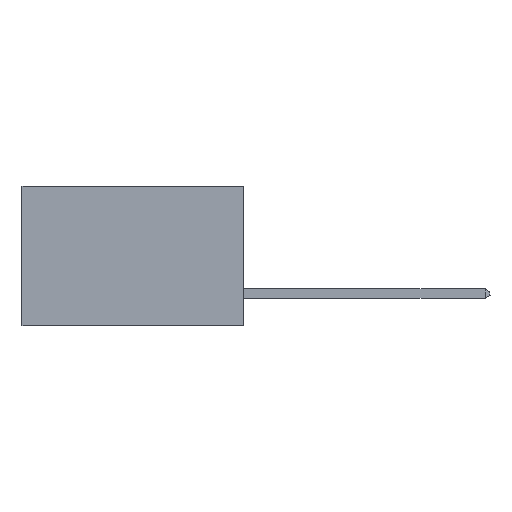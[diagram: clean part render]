
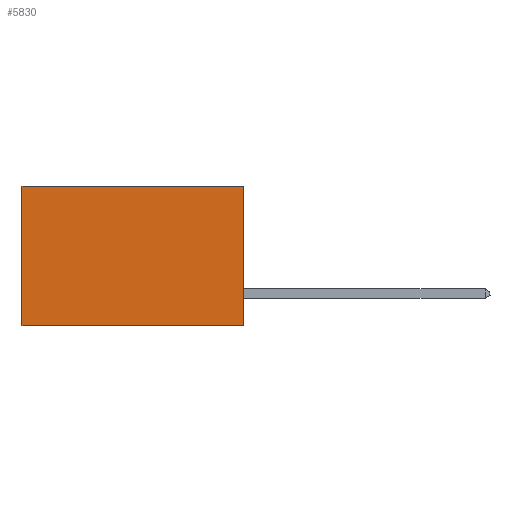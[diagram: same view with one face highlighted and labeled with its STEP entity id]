
A CAD part, left-side view. The second image highlights one B-rep face of the part: STEP entity #5830.
In plain terms, the highlighted planar face has unit normal (-1, 0, 0).
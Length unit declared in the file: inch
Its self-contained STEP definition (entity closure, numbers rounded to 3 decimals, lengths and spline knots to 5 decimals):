
#313 = VERTEX_POINT ( 'NONE', #10428 ) ;
#1306 = EDGE_LOOP ( 'NONE', ( #21295, #5080, #8119, #3326 ) ) ;
#1521 = VECTOR ( 'NONE', #9994, 39.37008 ) ;
#2545 = CARTESIAN_POINT ( 'NONE',  ( 0.277, 0.59, -0.37 ) ) ;
#3247 = CARTESIAN_POINT ( 'NONE',  ( 0.277, 0., 0. ) ) ;
#3326 = ORIENTED_EDGE ( 'NONE', *, *, #8300, .T. ) ;
#4000 = VECTOR ( 'NONE', #4506, 39.37008 ) ;
#4055 = EDGE_CURVE ( 'NONE', #6846, #10834, #22341, .T. ) ;
#4356 = CARTESIAN_POINT ( 'NONE',  ( 0.277, 0., -0.37 ) ) ;
#4506 = DIRECTION ( 'NONE',  ( 0., 0., -1. ) ) ;
#5080 = ORIENTED_EDGE ( 'NONE', *, *, #6585, .F. ) ;
#5112 = FACE_OUTER_BOUND ( 'NONE', #1306, .T. ) ;
#5409 = AXIS2_PLACEMENT_3D ( 'NONE', #12770, #12705, #12666 ) ;
#5830 = ADVANCED_FACE ( 'NONE', ( #5112 ), #13014, .F. ) ;
#6585 = EDGE_CURVE ( 'NONE', #10834, #313, #7511, .T. ) ;
#6846 = VERTEX_POINT ( 'NONE', #3247 ) ;
#7511 = LINE ( 'NONE', #11768, #22531 ) ;
#8119 = ORIENTED_EDGE ( 'NONE', *, *, #4055, .F. ) ;
#8300 = EDGE_CURVE ( 'NONE', #6846, #14964, #15487, .T. ) ;
#9211 = LINE ( 'NONE', #2545, #4000 ) ;
#9491 = DIRECTION ( 'NONE',  ( 0., 1., 0. ) ) ;
#9542 = CARTESIAN_POINT ( 'NONE',  ( 0.277, 0., 0. ) ) ;
#9994 = DIRECTION ( 'NONE',  ( 0., 0., -1. ) ) ;
#10407 = CARTESIAN_POINT ( 'NONE',  ( 0.277, 0., -0.37 ) ) ;
#10428 = CARTESIAN_POINT ( 'NONE',  ( 0.277, 0.59, -0.37 ) ) ;
#10834 = VERTEX_POINT ( 'NONE', #4356 ) ;
#11768 = CARTESIAN_POINT ( 'NONE',  ( 0.277, 0., -0.37 ) ) ;
#11796 = DIRECTION ( 'NONE',  ( 0., 1., 0. ) ) ;
#12666 = DIRECTION ( 'NONE',  ( 0., 0., -1. ) ) ;
#12705 = DIRECTION ( 'NONE',  ( 1., 0., 0. ) ) ;
#12770 = CARTESIAN_POINT ( 'NONE',  ( 0.277, 0., -0.37 ) ) ;
#13014 = PLANE ( 'NONE',  #5409 ) ;
#13069 = CARTESIAN_POINT ( 'NONE',  ( 0.277, 0.59, 0. ) ) ;
#14878 = VECTOR ( 'NONE', #9491, 39.37008 ) ;
#14964 = VERTEX_POINT ( 'NONE', #13069 ) ;
#15487 = LINE ( 'NONE', #9542, #14878 ) ;
#21295 = ORIENTED_EDGE ( 'NONE', *, *, #23291, .T. ) ;
#22341 = LINE ( 'NONE', #10407, #1521 ) ;
#22531 = VECTOR ( 'NONE', #11796, 39.37008 ) ;
#23291 = EDGE_CURVE ( 'NONE', #14964, #313, #9211, .T. ) ;
